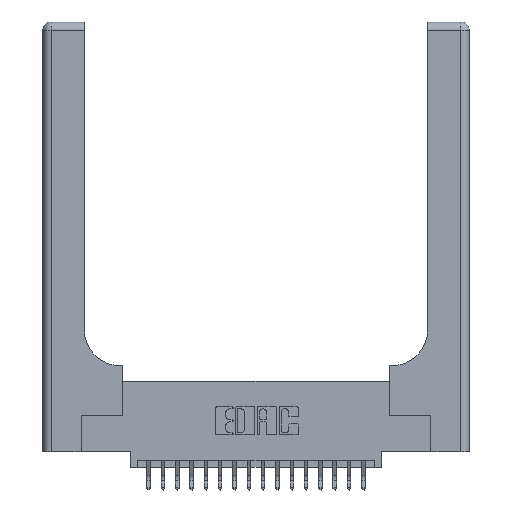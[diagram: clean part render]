
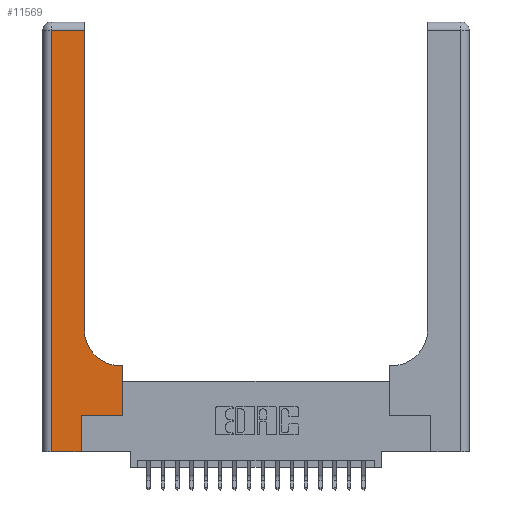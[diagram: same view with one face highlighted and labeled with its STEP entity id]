
A CAD part, top view. The second image highlights one B-rep face of the part: STEP entity #11569.
In plain terms, the highlighted planar face has unit normal (0, 0, 1).
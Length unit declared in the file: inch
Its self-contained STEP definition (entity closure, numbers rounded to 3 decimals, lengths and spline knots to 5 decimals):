
#385 = EDGE_CURVE ( 'NONE', #20675, #18656, #9619, .T. ) ;
#396 = EDGE_CURVE ( 'NONE', #8466, #4018, #10375, .T. ) ;
#411 = CARTESIAN_POINT ( 'NONE',  ( 0., 3., 0.37 ) ) ;
#785 = EDGE_LOOP ( 'NONE', ( #18797, #12464, #15404, #11066, #9531, #4644, #12521, #1442, #12056 ) ) ;
#1256 = DIRECTION ( 'NONE',  ( -1., 0., 0. ) ) ;
#1284 = VECTOR ( 'NONE', #17767, 39.37008 ) ;
#1442 = ORIENTED_EDGE ( 'NONE', *, *, #11910, .T. ) ;
#1518 = EDGE_CURVE ( 'NONE', #5392, #16481, #20504, .T. ) ;
#2042 = VECTOR ( 'NONE', #1256, 39.37008 ) ;
#2794 = CIRCLE ( 'NONE', #6823, 0.25 ) ;
#3461 = VECTOR ( 'NONE', #20183, 39.37008 ) ;
#3569 = CARTESIAN_POINT ( 'NONE',  ( 0.269, 0.25, 0.37 ) ) ;
#3623 = VECTOR ( 'NONE', #19590, 39.37008 ) ;
#4018 = VERTEX_POINT ( 'NONE', #20025 ) ;
#4130 = EDGE_CURVE ( 'NONE', #20085, #20675, #2794, .T. ) ;
#4644 = ORIENTED_EDGE ( 'NONE', *, *, #20136, .T. ) ;
#5124 = DIRECTION ( 'NONE',  ( -1., 0., 0. ) ) ;
#5392 = VERTEX_POINT ( 'NONE', #20018 ) ;
#6823 = AXIS2_PLACEMENT_3D ( 'NONE', #20331, #13746, #15350 ) ;
#7975 = LINE ( 'NONE', #20722, #9746 ) ;
#8466 = VERTEX_POINT ( 'NONE', #17141 ) ;
#8530 = EDGE_CURVE ( 'NONE', #16481, #8466, #16407, .T. ) ;
#8657 = EDGE_CURVE ( 'NONE', #18656, #5392, #10935, .T. ) ;
#9531 = ORIENTED_EDGE ( 'NONE', *, *, #396, .T. ) ;
#9619 = LINE ( 'NONE', #11216, #1284 ) ;
#9746 = VECTOR ( 'NONE', #20435, 39.37008 ) ;
#10375 = LINE ( 'NONE', #17924, #3623 ) ;
#10422 = CARTESIAN_POINT ( 'NONE',  ( 0.2915, 0.6, 0.37 ) ) ;
#10735 = LINE ( 'NONE', #3569, #3461 ) ;
#10754 = VECTOR ( 'NONE', #12171, 39.37008 ) ;
#10935 = LINE ( 'NONE', #12701, #2042 ) ;
#11066 = ORIENTED_EDGE ( 'NONE', *, *, #8530, .T. ) ;
#11093 = EDGE_CURVE ( 'NONE', #11999, #18946, #7975, .T. ) ;
#11216 = CARTESIAN_POINT ( 'NONE',  ( 0.2915, 3., 0.37 ) ) ;
#11387 = CARTESIAN_POINT ( 'NONE',  ( 0.5585, 0.6, 0.37 ) ) ;
#11569 = ADVANCED_FACE ( 'NONE', ( #15695 ), #13535, .F. ) ;
#11910 = EDGE_CURVE ( 'NONE', #18946, #20085, #13601, .T. ) ;
#11999 = VERTEX_POINT ( 'NONE', #19100 ) ;
#12056 = ORIENTED_EDGE ( 'NONE', *, *, #4130, .T. ) ;
#12159 = CARTESIAN_POINT ( 'NONE',  ( 0.2915, 2.94, 0.37 ) ) ;
#12171 = DIRECTION ( 'NONE',  ( -1., 0., 0. ) ) ;
#12464 = ORIENTED_EDGE ( 'NONE', *, *, #8657, .T. ) ;
#12521 = ORIENTED_EDGE ( 'NONE', *, *, #11093, .T. ) ;
#12701 = CARTESIAN_POINT ( 'NONE',  ( 0., 2.94, 0.37 ) ) ;
#13380 = CARTESIAN_POINT ( 'NONE',  ( 0.2915, 0.85, 0.37 ) ) ;
#13535 = PLANE ( 'NONE',  #19729 ) ;
#13601 = LINE ( 'NONE', #10422, #10754 ) ;
#13746 = DIRECTION ( 'NONE',  ( 0., 0., -1. ) ) ;
#15350 = DIRECTION ( 'NONE',  ( 1., 0., 0. ) ) ;
#15351 = DIRECTION ( 'NONE',  ( 0., -1., 0. ) ) ;
#15404 = ORIENTED_EDGE ( 'NONE', *, *, #1518, .T. ) ;
#15592 = DIRECTION ( 'NONE',  ( 1., 0., 0. ) ) ;
#15695 = FACE_OUTER_BOUND ( 'NONE', #785, .T. ) ;
#16364 = VECTOR ( 'NONE', #15351, 39.37008 ) ;
#16407 = LINE ( 'NONE', #17430, #20310 ) ;
#16481 = VERTEX_POINT ( 'NONE', #21614 ) ;
#16895 = CARTESIAN_POINT ( 'NONE',  ( 0.5415, 0.6, 0.37 ) ) ;
#17141 = CARTESIAN_POINT ( 'NONE',  ( 0.269, 0., 0.37 ) ) ;
#17430 = CARTESIAN_POINT ( 'NONE',  ( 0., 0., 0.37 ) ) ;
#17767 = DIRECTION ( 'NONE',  ( 0., 1., 0. ) ) ;
#17924 = CARTESIAN_POINT ( 'NONE',  ( 0.269, 0., 0.37 ) ) ;
#18656 = VERTEX_POINT ( 'NONE', #12159 ) ;
#18719 = DIRECTION ( 'NONE',  ( 0., 0., -1. ) ) ;
#18797 = ORIENTED_EDGE ( 'NONE', *, *, #385, .T. ) ;
#18946 = VERTEX_POINT ( 'NONE', #11387 ) ;
#19100 = CARTESIAN_POINT ( 'NONE',  ( 0.5585, 0.25, 0.37 ) ) ;
#19590 = DIRECTION ( 'NONE',  ( 0., 1., 0. ) ) ;
#19729 = AXIS2_PLACEMENT_3D ( 'NONE', #411, #18719, #5124 ) ;
#20018 = CARTESIAN_POINT ( 'NONE',  ( 0.06, 2.94, 0.37 ) ) ;
#20025 = CARTESIAN_POINT ( 'NONE',  ( 0.269, 0.25, 0.37 ) ) ;
#20085 = VERTEX_POINT ( 'NONE', #16895 ) ;
#20136 = EDGE_CURVE ( 'NONE', #4018, #11999, #10735, .T. ) ;
#20183 = DIRECTION ( 'NONE',  ( 1., 0., 0. ) ) ;
#20310 = VECTOR ( 'NONE', #15592, 39.37008 ) ;
#20331 = CARTESIAN_POINT ( 'NONE',  ( 0.5415, 0.85, 0.37 ) ) ;
#20435 = DIRECTION ( 'NONE',  ( 0., 1., 0. ) ) ;
#20504 = LINE ( 'NONE', #20534, #16364 ) ;
#20534 = CARTESIAN_POINT ( 'NONE',  ( 0.06, 3., 0.37 ) ) ;
#20675 = VERTEX_POINT ( 'NONE', #13380 ) ;
#20722 = CARTESIAN_POINT ( 'NONE',  ( 0.5585, 0.25, 0.37 ) ) ;
#21614 = CARTESIAN_POINT ( 'NONE',  ( 0.06, 0., 0.37 ) ) ;
